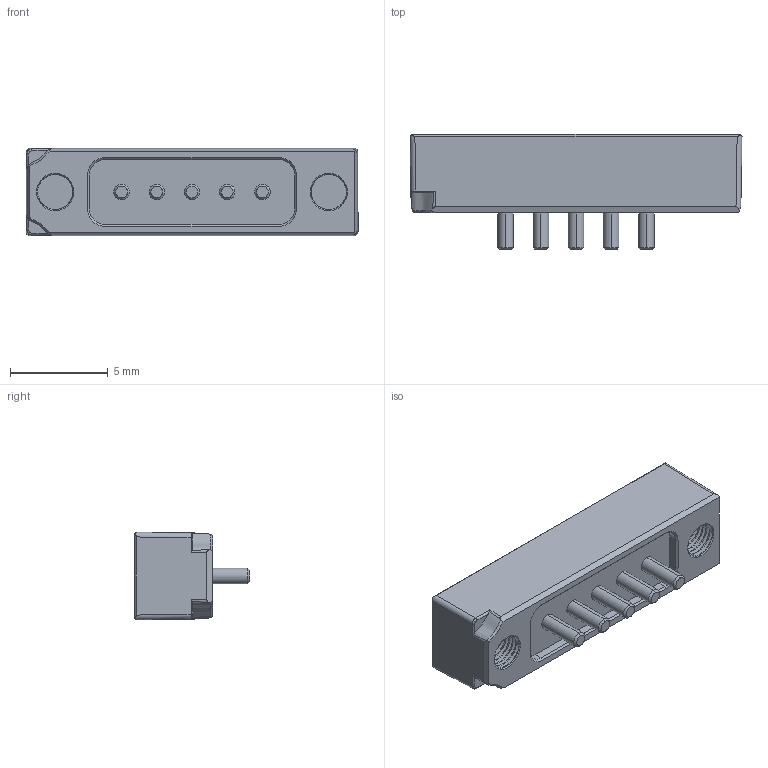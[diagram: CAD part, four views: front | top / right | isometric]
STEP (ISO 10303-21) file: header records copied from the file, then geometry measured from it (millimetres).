
FILE_DESCRIPTION (( 'STEP AP214' ), '1' );
FILE_NAME ('686B0521410117E.STEP', '2023-05-01T19:28:46', ( '' ), ( '' ), 'SwSTEP 2.0', 'SolidWorks 2020', '' );
FILE_SCHEMA (( 'AUTOMOTIVE_DESIGN' ));
Length unit declared in the file: millimetre
Products named in the file (1): 686B0521410117E
Bounding box: 16.99 x 5.9 x 4.5 mm (x, y, z)
Volume: 249.6 mm3; surface area: 449.9 mm2
Topology: 1 solids, 1 shells, 184 faces, 452 edges, 284 vertices
Faces by surface type: cylinder 84, plane 50, cone 32, bspline 18
Entity records: 10098 total; most frequent: CARTESIAN_POINT 4173, ORIENTED_EDGE 904, DIRECTION 748, EDGE_CURVE 452, VERTEX_POINT 284, AXIS2_PLACEMENT_3D 275, LINE 198, EDGE_LOOP 198
